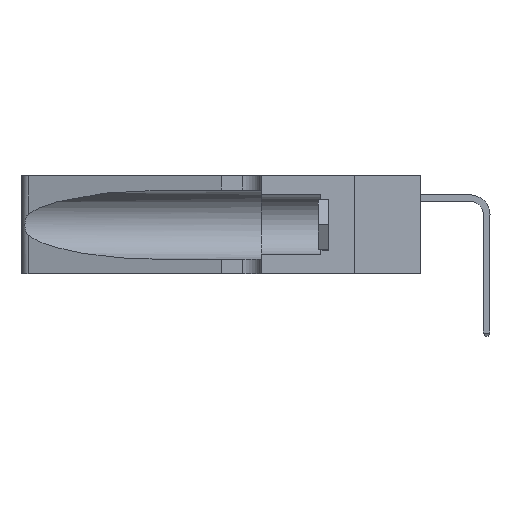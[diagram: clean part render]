
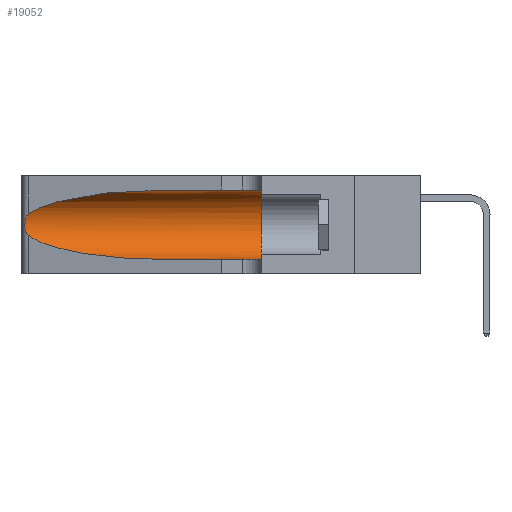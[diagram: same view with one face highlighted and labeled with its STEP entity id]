
A CAD part, left-side view. The second image highlights one B-rep face of the part: STEP entity #19052.
In plain terms, the highlighted cylindrical face has radius 3.308 mm (diameter 6.617 mm), a partial arc.
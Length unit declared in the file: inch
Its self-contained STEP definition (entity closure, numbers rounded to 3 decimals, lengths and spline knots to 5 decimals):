
#24 = FACE_OUTER_BOUND ( 'NONE', #24157, .T. ) ;
#218 =( BOUNDED_CURVE ( )  B_SPLINE_CURVE ( 3, ( #11776, #16118, #5392, #20418 ),
 .UNSPECIFIED., .F., .F. ) 
 B_SPLINE_CURVE_WITH_KNOTS ( ( 4, 4 ),
 ( 3.44316, 4.71239 ),
 .UNSPECIFIED. ) 
 CURVE ( )  GEOMETRIC_REPRESENTATION_ITEM ( )  RATIONAL_B_SPLINE_CURVE ( ( 1., 0.87, 0.87, 1. ) ) 
 REPRESENTATION_ITEM ( '' )  );
#555 = CARTESIAN_POINT ( 'NONE',  ( 0.1305, 0.72297, 0.31525 ) ) ;
#1023 = DIRECTION ( 'NONE',  ( 0., 0., -1. ) ) ;
#1624 = CARTESIAN_POINT ( 'NONE',  ( 0.25787, 1.23484, 0.2124 ) ) ;
#1692 = VERTEX_POINT ( 'NONE', #8513 ) ;
#3410 = CARTESIAN_POINT ( 'NONE',  ( 0.1305, 1.61858, 0.05475 ) ) ;
#3743 = CARTESIAN_POINT ( 'NONE',  ( 0.26018, 1.23835, 0.19895 ) ) ;
#3905 = DIRECTION ( 'NONE',  ( 0., -1., 0. ) ) ;
#4783 = DIRECTION ( 'NONE',  ( 0., 1., 0. ) ) ;
#4850 = EDGE_CURVE ( 'NONE', #23480, #27370, #15164, .T. ) ;
#5186 = B_SPLINE_CURVE_WITH_KNOTS ( 'NONE', 3,
 ( #25091, #27200, #14411, #1624, #16623, #3743, #18781, #5881, #20915, #8008, #23041, #10161, #25184, #12365 ),
 .UNSPECIFIED., .F., .F.,
 ( 4, 2, 2, 2, 2, 2, 4 ),
 ( 0., 0.00027, 0.00053, 0.00107, 0.0016, 0.00187, 0.00214 ),
 .UNSPECIFIED. ) ;
#5392 = CARTESIAN_POINT ( 'NONE',  ( 0.18966, 0.96281, 0.05475 ) ) ;
#5881 = CARTESIAN_POINT ( 'NONE',  ( 0.26075, 1.23896, 0.178 ) ) ;
#6544 = ORIENTED_EDGE ( 'NONE', *, *, #9710, .T. ) ;
#7426 = CARTESIAN_POINT ( 'NONE',  ( 0.1305, 1.61858, 0.185 ) ) ;
#8008 = CARTESIAN_POINT ( 'NONE',  ( 0.25856, 1.23593, 0.16098 ) ) ;
#8183 = VERTEX_POINT ( 'NONE', #24991 ) ;
#8238 = EDGE_CURVE ( 'NONE', #23480, #8183, #27182, .T. ) ;
#8513 = CARTESIAN_POINT ( 'NONE',  ( 0.25487, 1.22718, 0.14631 ) ) ;
#8577 = CIRCLE ( 'NONE', #23895, 0.13025 ) ;
#9350 = CYLINDRICAL_SURFACE ( 'NONE', #22493, 0.13025 ) ;
#9422 = VECTOR ( 'NONE', #3905, 39.37008 ) ;
#9496 = CARTESIAN_POINT ( 'NONE',  ( 0.1305, 0.72297, 0.05475 ) ) ;
#9710 = EDGE_CURVE ( 'NONE', #27370, #1692, #5186, .T. ) ;
#10161 = CARTESIAN_POINT ( 'NONE',  ( 0.25639, 1.23186, 0.15144 ) ) ;
#10181 = EDGE_CURVE ( 'NONE', #1692, #11796, #218, .T. ) ;
#11192 = CARTESIAN_POINT ( 'NONE',  ( 0.18966, 0.96281, 0.31525 ) ) ;
#11310 = EDGE_CURVE ( 'NONE', #8183, #18566, #8577, .T. ) ;
#11672 = DIRECTION ( 'NONE',  ( 0., -1., 0. ) ) ;
#11776 = CARTESIAN_POINT ( 'NONE',  ( 0.25487, 1.22718, 0.14631 ) ) ;
#11796 = VERTEX_POINT ( 'NONE', #9496 ) ;
#12365 = CARTESIAN_POINT ( 'NONE',  ( 0.25487, 1.22718, 0.14631 ) ) ;
#13489 = LINE ( 'NONE', #3410, #24203 ) ;
#13602 = ORIENTED_EDGE ( 'NONE', *, *, #8238, .F. ) ;
#14082 = CARTESIAN_POINT ( 'NONE',  ( 0.25487, 1.22718, 0.22369 ) ) ;
#14160 = DIRECTION ( 'NONE',  ( 0., -1., 0. ) ) ;
#14249 = CARTESIAN_POINT ( 'NONE',  ( 0.1305, 0.72297, 0.31525 ) ) ;
#14411 = CARTESIAN_POINT ( 'NONE',  ( 0.25639, 1.23184, 0.21858 ) ) ;
#15164 =( BOUNDED_CURVE ( )  B_SPLINE_CURVE ( 3, ( #555, #11192, #19755, #15549 ),
 .UNSPECIFIED., .F., .T. ) 
 B_SPLINE_CURVE_WITH_KNOTS ( ( 4, 4 ),
 ( 1.5708, 2.84003 ),
 .UNSPECIFIED. ) 
 CURVE ( )  GEOMETRIC_REPRESENTATION_ITEM ( )  RATIONAL_B_SPLINE_CURVE ( ( 1., 0.87, 0.87, 1. ) ) 
 REPRESENTATION_ITEM ( '' )  );
#15549 = CARTESIAN_POINT ( 'NONE',  ( 0.25487, 1.22718, 0.22369 ) ) ;
#16118 = CARTESIAN_POINT ( 'NONE',  ( 0.2373, 1.15595, 0.08982 ) ) ;
#16623 = CARTESIAN_POINT ( 'NONE',  ( 0.25854, 1.2359, 0.20912 ) ) ;
#16779 = CARTESIAN_POINT ( 'NONE',  ( 0.1305, 1.61858, 0.31525 ) ) ;
#17667 = CARTESIAN_POINT ( 'NONE',  ( 0.1305, 0.35, 0.185 ) ) ;
#18051 = EDGE_CURVE ( 'NONE', #11796, #18566, #13489, .T. ) ;
#18566 = VERTEX_POINT ( 'NONE', #22485 ) ;
#18781 = CARTESIAN_POINT ( 'NONE',  ( 0.26075, 1.23896, 0.19203 ) ) ;
#19052 = ADVANCED_FACE ( 'NONE', ( #24 ), #9350, .F. ) ;
#19755 = CARTESIAN_POINT ( 'NONE',  ( 0.2373, 1.15595, 0.28018 ) ) ;
#19785 = DIRECTION ( 'NONE',  ( 0., 0., 1. ) ) ;
#20418 = CARTESIAN_POINT ( 'NONE',  ( 0.1305, 0.72297, 0.05475 ) ) ;
#20859 = ORIENTED_EDGE ( 'NONE', *, *, #4850, .T. ) ;
#20915 = CARTESIAN_POINT ( 'NONE',  ( 0.26017, 1.23833, 0.17102 ) ) ;
#21555 = ORIENTED_EDGE ( 'NONE', *, *, #11310, .F. ) ;
#22485 = CARTESIAN_POINT ( 'NONE',  ( 0.1305, 0.35, 0.05475 ) ) ;
#22493 = AXIS2_PLACEMENT_3D ( 'NONE', #7426, #11672, #1023 ) ;
#22909 = ORIENTED_EDGE ( 'NONE', *, *, #10181, .T. ) ;
#23041 = CARTESIAN_POINT ( 'NONE',  ( 0.25789, 1.23486, 0.15765 ) ) ;
#23294 = ORIENTED_EDGE ( 'NONE', *, *, #18051, .T. ) ;
#23480 = VERTEX_POINT ( 'NONE', #14249 ) ;
#23895 = AXIS2_PLACEMENT_3D ( 'NONE', #17667, #4783, #19785 ) ;
#24157 = EDGE_LOOP ( 'NONE', ( #20859, #6544, #22909, #23294, #21555, #13602 ) ) ;
#24203 = VECTOR ( 'NONE', #14160, 39.37008 ) ;
#24991 = CARTESIAN_POINT ( 'NONE',  ( 0.1305, 0.35, 0.31525 ) ) ;
#25091 = CARTESIAN_POINT ( 'NONE',  ( 0.25487, 1.22718, 0.22369 ) ) ;
#25184 = CARTESIAN_POINT ( 'NONE',  ( 0.25555, 1.22993, 0.14849 ) ) ;
#27182 = LINE ( 'NONE', #16779, #9422 ) ;
#27200 = CARTESIAN_POINT ( 'NONE',  ( 0.25555, 1.22994, 0.2215 ) ) ;
#27370 = VERTEX_POINT ( 'NONE', #14082 ) ;
